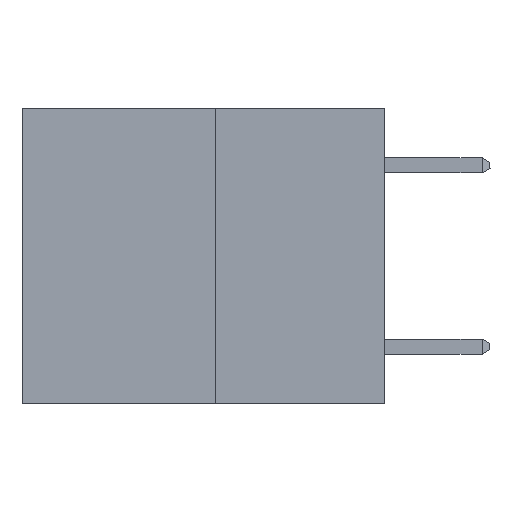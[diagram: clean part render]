
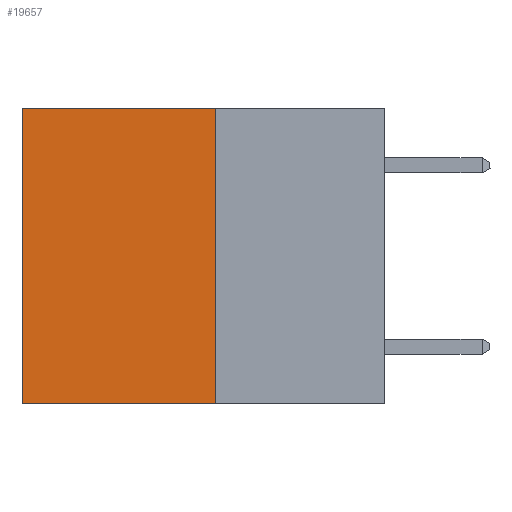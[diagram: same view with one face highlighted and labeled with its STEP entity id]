
A CAD part, left-side view. The second image highlights one B-rep face of the part: STEP entity #19657.
In plain terms, the highlighted planar face has unit normal (-1, 0, 0).
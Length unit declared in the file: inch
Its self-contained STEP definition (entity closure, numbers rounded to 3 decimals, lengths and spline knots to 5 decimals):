
#235 = ORIENTED_EDGE ( 'NONE', *, *, #2189, .T. ) ;
#1274 = EDGE_CURVE ( 'NONE', #8707, #9936, #10794, .T. ) ;
#1639 = ORIENTED_EDGE ( 'NONE', *, *, #14307, .F. ) ;
#2189 = EDGE_CURVE ( 'NONE', #7375, #9360, #15404, .T. ) ;
#2514 = VECTOR ( 'NONE', #4628, 39.37008 ) ;
#3203 = LINE ( 'NONE', #6798, #17411 ) ;
#4385 = CARTESIAN_POINT ( 'NONE',  ( 0.3165, 0.6, -0.49 ) ) ;
#4480 = CARTESIAN_POINT ( 'NONE',  ( 0.3165, 0.28, -0.49 ) ) ;
#4628 = DIRECTION ( 'NONE',  ( 0., 0., -1. ) ) ;
#5991 = CARTESIAN_POINT ( 'NONE',  ( 0.3165, 0.28, 0. ) ) ;
#6734 = DIRECTION ( 'NONE',  ( 0., 1., 0. ) ) ;
#6798 = CARTESIAN_POINT ( 'NONE',  ( 0.3165, 0.28, -0.49 ) ) ;
#6972 = ORIENTED_EDGE ( 'NONE', *, *, #13719, .T. ) ;
#7375 = VERTEX_POINT ( 'NONE', #17613 ) ;
#7703 = CARTESIAN_POINT ( 'NONE',  ( 0.3165, 0.28, 0. ) ) ;
#8595 = DIRECTION ( 'NONE',  ( 0., 0., -1. ) ) ;
#8707 = VERTEX_POINT ( 'NONE', #5991 ) ;
#9360 = VERTEX_POINT ( 'NONE', #4385 ) ;
#9885 = PLANE ( 'NONE',  #15139 ) ;
#9936 = VERTEX_POINT ( 'NONE', #16408 ) ;
#10425 = LINE ( 'NONE', #7703, #20771 ) ;
#10794 = LINE ( 'NONE', #4480, #2514 ) ;
#11038 = DIRECTION ( 'NONE',  ( 0., 0., -1. ) ) ;
#12761 = DIRECTION ( 'NONE',  ( 1., 0., 0. ) ) ;
#13173 = DIRECTION ( 'NONE',  ( 0., 1., 0. ) ) ;
#13719 = EDGE_CURVE ( 'NONE', #8707, #7375, #10425, .T. ) ;
#14307 = EDGE_CURVE ( 'NONE', #9936, #9360, #3203, .T. ) ;
#15117 = ORIENTED_EDGE ( 'NONE', *, *, #1274, .F. ) ;
#15139 = AXIS2_PLACEMENT_3D ( 'NONE', #17680, #12761, #11038 ) ;
#15404 = LINE ( 'NONE', #18467, #20323 ) ;
#16408 = CARTESIAN_POINT ( 'NONE',  ( 0.3165, 0.28, -0.49 ) ) ;
#17066 = EDGE_LOOP ( 'NONE', ( #235, #1639, #15117, #6972 ) ) ;
#17411 = VECTOR ( 'NONE', #6734, 39.37008 ) ;
#17613 = CARTESIAN_POINT ( 'NONE',  ( 0.3165, 0.6, 0. ) ) ;
#17680 = CARTESIAN_POINT ( 'NONE',  ( 0.3165, 0.28, -0.49 ) ) ;
#18467 = CARTESIAN_POINT ( 'NONE',  ( 0.3165, 0.6, -0.49 ) ) ;
#19156 = FACE_OUTER_BOUND ( 'NONE', #17066, .T. ) ;
#19657 = ADVANCED_FACE ( 'NONE', ( #19156 ), #9885, .F. ) ;
#20323 = VECTOR ( 'NONE', #8595, 39.37008 ) ;
#20771 = VECTOR ( 'NONE', #13173, 39.37008 ) ;
